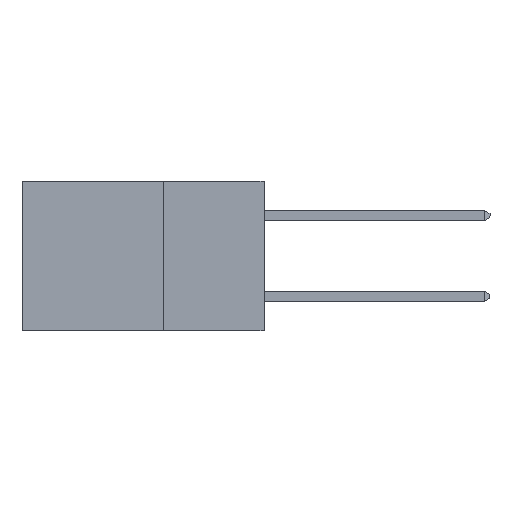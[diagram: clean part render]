
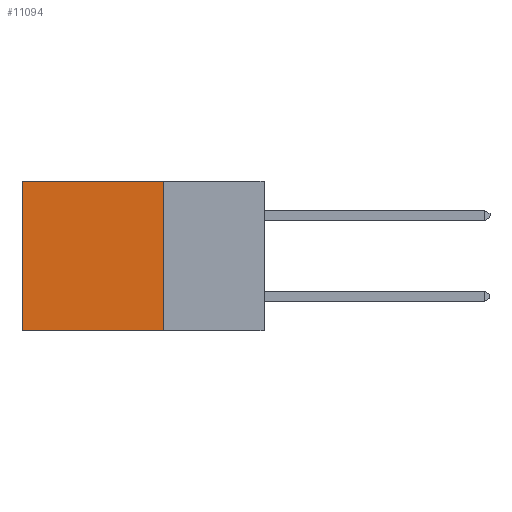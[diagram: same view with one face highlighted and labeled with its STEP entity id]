
A CAD part, left-side view. The second image highlights one B-rep face of the part: STEP entity #11094.
In plain terms, the highlighted planar face has unit normal (-1, 0, 0).
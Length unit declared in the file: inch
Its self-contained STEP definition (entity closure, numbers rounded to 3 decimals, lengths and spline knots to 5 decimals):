
#85 = ORIENTED_EDGE ( 'NONE', *, *, #2693, .F. ) ;
#290 = AXIS2_PLACEMENT_3D ( 'NONE', #10142, #10936, #5821 ) ;
#859 = CARTESIAN_POINT ( 'NONE',  ( 0.298, 0.25, 0. ) ) ;
#1265 = FACE_OUTER_BOUND ( 'NONE', #5455, .T. ) ;
#1294 = PLANE ( 'NONE',  #290 ) ;
#2061 = VERTEX_POINT ( 'NONE', #4547 ) ;
#2282 = VERTEX_POINT ( 'NONE', #2775 ) ;
#2435 = EDGE_CURVE ( 'NONE', #2282, #2061, #10747, .T. ) ;
#2693 = EDGE_CURVE ( 'NONE', #2282, #3144, #10624, .T. ) ;
#2775 = CARTESIAN_POINT ( 'NONE',  ( 0.298, 0.25, 0. ) ) ;
#2872 = CARTESIAN_POINT ( 'NONE',  ( 0.298, 0.25, -0.37 ) ) ;
#2944 = VERTEX_POINT ( 'NONE', #4655 ) ;
#3144 = VERTEX_POINT ( 'NONE', #4854 ) ;
#3627 = EDGE_CURVE ( 'NONE', #2061, #2944, #10863, .T. ) ;
#3794 = LINE ( 'NONE', #2872, #5852 ) ;
#4014 = VECTOR ( 'NONE', #9224, 39.37008 ) ;
#4547 = CARTESIAN_POINT ( 'NONE',  ( 0.298, 0.6, 0. ) ) ;
#4655 = CARTESIAN_POINT ( 'NONE',  ( 0.298, 0.6, -0.37 ) ) ;
#4854 = CARTESIAN_POINT ( 'NONE',  ( 0.298, 0.25, -0.37 ) ) ;
#5455 = EDGE_LOOP ( 'NONE', ( #8892, #5549, #85, #11023 ) ) ;
#5549 = ORIENTED_EDGE ( 'NONE', *, *, #10843, .F. ) ;
#5646 = DIRECTION ( 'NONE',  ( 0., 0., -1. ) ) ;
#5821 = DIRECTION ( 'NONE',  ( 0., 0., -1. ) ) ;
#5852 = VECTOR ( 'NONE', #8220, 39.37008 ) ;
#8173 = VECTOR ( 'NONE', #5646, 39.37008 ) ;
#8220 = DIRECTION ( 'NONE',  ( 0., 1., 0. ) ) ;
#8892 = ORIENTED_EDGE ( 'NONE', *, *, #3627, .T. ) ;
#9122 = CARTESIAN_POINT ( 'NONE',  ( 0.298, 0.25, 0. ) ) ;
#9224 = DIRECTION ( 'NONE',  ( 0., 0., -1. ) ) ;
#9690 = DIRECTION ( 'NONE',  ( 0., 1., 0. ) ) ;
#10142 = CARTESIAN_POINT ( 'NONE',  ( 0.298, 0.25, 0. ) ) ;
#10162 = CARTESIAN_POINT ( 'NONE',  ( 0.298, 0.6, 0. ) ) ;
#10624 = LINE ( 'NONE', #9122, #8173 ) ;
#10747 = LINE ( 'NONE', #859, #11003 ) ;
#10843 = EDGE_CURVE ( 'NONE', #3144, #2944, #3794, .T. ) ;
#10863 = LINE ( 'NONE', #10162, #4014 ) ;
#10936 = DIRECTION ( 'NONE',  ( 1., 0., 0. ) ) ;
#11003 = VECTOR ( 'NONE', #9690, 39.37008 ) ;
#11023 = ORIENTED_EDGE ( 'NONE', *, *, #2435, .T. ) ;
#11094 = ADVANCED_FACE ( 'NONE', ( #1265 ), #1294, .F. ) ;
